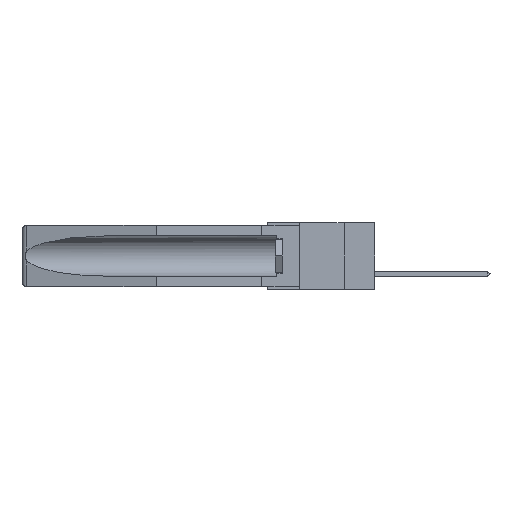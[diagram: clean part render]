
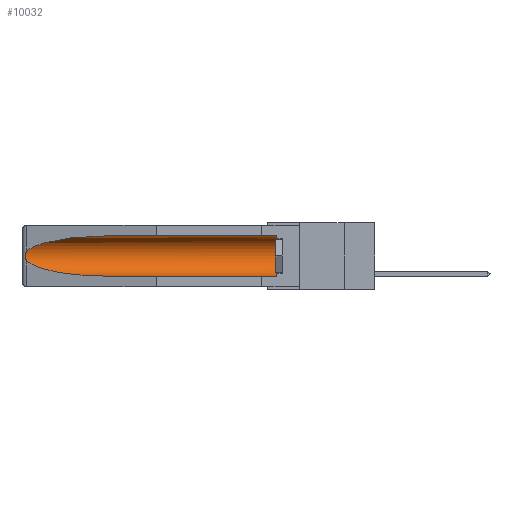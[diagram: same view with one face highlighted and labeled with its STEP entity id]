
A CAD part, left-side view. The second image highlights one B-rep face of the part: STEP entity #10032.
In plain terms, the highlighted cylindrical face has radius 2.857 mm (diameter 5.715 mm), a partial arc.
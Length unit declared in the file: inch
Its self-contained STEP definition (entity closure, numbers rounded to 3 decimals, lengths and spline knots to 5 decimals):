
#178 = CARTESIAN_POINT ( 'NONE',  ( 0.26537, 1.52718, -0.14972 ) ) ;
#217 = AXIS2_PLACEMENT_3D ( 'NONE', #1312, #13137, #5793 ) ;
#359 =( BOUNDED_CURVE ( )  B_SPLINE_CURVE ( 3, ( #13479, #17898, #9159, #178 ),
 .UNSPECIFIED., .F., .F. ) 
 B_SPLINE_CURVE_WITH_KNOTS ( ( 4, 4 ),
 ( 4.71239, 6.08839 ),
 .UNSPECIFIED. ) 
 CURVE ( )  GEOMETRIC_REPRESENTATION_ITEM ( )  RATIONAL_B_SPLINE_CURVE ( ( 1., 0.848, 0.848, 1. ) ) 
 REPRESENTATION_ITEM ( '' )  );
#546 = CARTESIAN_POINT ( 'NONE',  ( 0.21114, 1.30732, -0.284 ) ) ;
#847 = VERTEX_POINT ( 'NONE', #1631 ) ;
#929 = ORIENTED_EDGE ( 'NONE', *, *, #2594, .T. ) ;
#1104 = VERTEX_POINT ( 'NONE', #18487 ) ;
#1312 = CARTESIAN_POINT ( 'NONE',  ( 0.155, -0.30754, -0.1715 ) ) ;
#1371 = CARTESIAN_POINT ( 'NONE',  ( 0.155, -0.30754, -0.284 ) ) ;
#1506 = LINE ( 'NONE', #1371, #4340 ) ;
#1631 = CARTESIAN_POINT ( 'NONE',  ( 0.26537, 1.52718, -0.14972 ) ) ;
#2128 = CARTESIAN_POINT ( 'NONE',  ( 0.26655, 1.53094, -0.18657 ) ) ;
#2594 = EDGE_CURVE ( 'NONE', #18597, #6607, #6433, .T. ) ;
#2842 = CARTESIAN_POINT ( 'NONE',  ( 0.155, 0.126, -0.284 ) ) ;
#3615 = CARTESIAN_POINT ( 'NONE',  ( 0.2675, 1.53308, -0.17534 ) ) ;
#4118 = CARTESIAN_POINT ( 'NONE',  ( 0.155, 0.126, -0.059 ) ) ;
#4340 = VECTOR ( 'NONE', #8967, 39.37008 ) ;
#4523 = CIRCLE ( 'NONE', #13663, 0.1125 ) ;
#4790 = CARTESIAN_POINT ( 'NONE',  ( 0.155, 1.07973, -0.284 ) ) ;
#5793 = DIRECTION ( 'NONE',  ( 0., 0., 1. ) ) ;
#6046 = EDGE_CURVE ( 'NONE', #1104, #847, #359, .T. ) ;
#6433 =( BOUNDED_CURVE ( )  B_SPLINE_CURVE ( 3, ( #10755, #15225, #546, #12369 ),
 .UNSPECIFIED., .F., .F. ) 
 B_SPLINE_CURVE_WITH_KNOTS ( ( 4, 4 ),
 ( 0.1948, 1.5708 ),
 .UNSPECIFIED. ) 
 CURVE ( )  GEOMETRIC_REPRESENTATION_ITEM ( )  RATIONAL_B_SPLINE_CURVE ( ( 1., 0.848, 0.848, 1. ) ) 
 REPRESENTATION_ITEM ( '' )  );
#6607 = VERTEX_POINT ( 'NONE', #4790 ) ;
#6673 = CARTESIAN_POINT ( 'NONE',  ( 0.26537, 1.52718, -0.19328 ) ) ;
#6696 = CARTESIAN_POINT ( 'NONE',  ( 0.2673, 1.5327, -0.16383 ) ) ;
#6715 = EDGE_LOOP ( 'NONE', ( #10401, #10494, #929, #7542, #11689, #10251 ) ) ;
#7542 = ORIENTED_EDGE ( 'NONE', *, *, #15546, .F. ) ;
#7834 = VERTEX_POINT ( 'NONE', #2842 ) ;
#8099 = DIRECTION ( 'NONE',  ( 0., -1., 0. ) ) ;
#8401 = B_SPLINE_CURVE_WITH_KNOTS ( 'NONE', 3,
 ( #9493, #12546, #11120, #6696, #16942, #3615, #14481, #2128, #12274, #17432 ),
 .UNSPECIFIED., .F., .F.,
 ( 4, 2, 2, 2, 4 ),
 ( 0., 0.00029, 0.00058, 0.00087, 0.00117 ),
 .UNSPECIFIED. ) ;
#8967 = DIRECTION ( 'NONE',  ( 0., 1., 0. ) ) ;
#9159 = CARTESIAN_POINT ( 'NONE',  ( 0.25451, 1.48313, -0.09465 ) ) ;
#9493 = CARTESIAN_POINT ( 'NONE',  ( 0.26537, 1.52718, -0.14972 ) ) ;
#10032 = ADVANCED_FACE ( 'NONE', ( #12256 ), #13845, .F. ) ;
#10251 = ORIENTED_EDGE ( 'NONE', *, *, #16834, .T. ) ;
#10401 = ORIENTED_EDGE ( 'NONE', *, *, #6046, .T. ) ;
#10494 = ORIENTED_EDGE ( 'NONE', *, *, #14733, .T. ) ;
#10718 = VECTOR ( 'NONE', #16044, 39.37008 ) ;
#10755 = CARTESIAN_POINT ( 'NONE',  ( 0.26537, 1.52718, -0.19328 ) ) ;
#11120 = CARTESIAN_POINT ( 'NONE',  ( 0.26654, 1.53092, -0.15636 ) ) ;
#11689 = ORIENTED_EDGE ( 'NONE', *, *, #16737, .T. ) ;
#12256 = FACE_OUTER_BOUND ( 'NONE', #6715, .T. ) ;
#12274 = CARTESIAN_POINT ( 'NONE',  ( 0.26597, 1.5296, -0.19026 ) ) ;
#12369 = CARTESIAN_POINT ( 'NONE',  ( 0.155, 1.07973, -0.284 ) ) ;
#12546 = CARTESIAN_POINT ( 'NONE',  ( 0.26597, 1.52961, -0.15275 ) ) ;
#12572 = LINE ( 'NONE', #14471, #10718 ) ;
#12753 = CARTESIAN_POINT ( 'NONE',  ( 0.155, 0.126, -0.1715 ) ) ;
#13137 = DIRECTION ( 'NONE',  ( 0., 1., 0. ) ) ;
#13410 = VERTEX_POINT ( 'NONE', #4118 ) ;
#13479 = CARTESIAN_POINT ( 'NONE',  ( 0.155, 1.07973, -0.059 ) ) ;
#13663 = AXIS2_PLACEMENT_3D ( 'NONE', #12753, #8099, #15666 ) ;
#13845 = CYLINDRICAL_SURFACE ( 'NONE', #217, 0.1125 ) ;
#14471 = CARTESIAN_POINT ( 'NONE',  ( 0.155, -0.30754, -0.059 ) ) ;
#14481 = CARTESIAN_POINT ( 'NONE',  ( 0.2673, 1.53269, -0.17917 ) ) ;
#14733 = EDGE_CURVE ( 'NONE', #847, #18597, #8401, .T. ) ;
#15225 = CARTESIAN_POINT ( 'NONE',  ( 0.25451, 1.48313, -0.24835 ) ) ;
#15546 = EDGE_CURVE ( 'NONE', #7834, #6607, #1506, .T. ) ;
#15666 = DIRECTION ( 'NONE',  ( 0., 0., 1. ) ) ;
#16044 = DIRECTION ( 'NONE',  ( 0., 1., 0. ) ) ;
#16737 = EDGE_CURVE ( 'NONE', #7834, #13410, #4523, .T. ) ;
#16834 = EDGE_CURVE ( 'NONE', #13410, #1104, #12572, .T. ) ;
#16942 = CARTESIAN_POINT ( 'NONE',  ( 0.2675, 1.53308, -0.16763 ) ) ;
#17432 = CARTESIAN_POINT ( 'NONE',  ( 0.26537, 1.52718, -0.19328 ) ) ;
#17898 = CARTESIAN_POINT ( 'NONE',  ( 0.21114, 1.30732, -0.059 ) ) ;
#18487 = CARTESIAN_POINT ( 'NONE',  ( 0.155, 1.07973, -0.059 ) ) ;
#18597 = VERTEX_POINT ( 'NONE', #6673 ) ;
